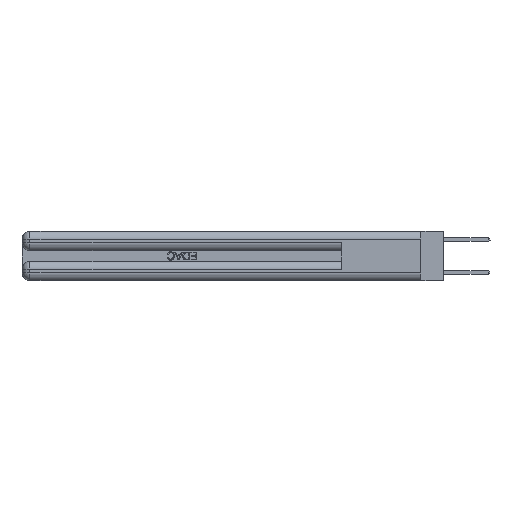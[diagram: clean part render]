
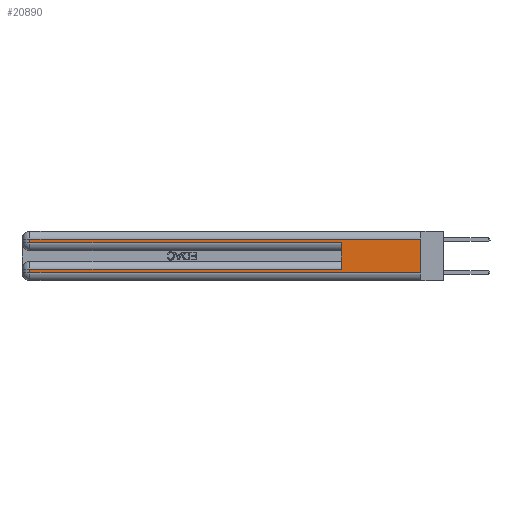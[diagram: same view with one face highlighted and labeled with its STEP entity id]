
A CAD part, left-side view. The second image highlights one B-rep face of the part: STEP entity #20890.
In plain terms, the highlighted planar face has unit normal (-1, 0, 0).
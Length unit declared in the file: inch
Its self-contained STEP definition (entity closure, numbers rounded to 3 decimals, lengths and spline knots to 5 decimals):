
#83 = LINE ( 'NONE', #20551, #28086 ) ;
#245 = LINE ( 'NONE', #5328, #17323 ) ;
#527 = CARTESIAN_POINT ( 'NONE',  ( 0., 2.94, 0.285 ) ) ;
#926 = DIRECTION ( 'NONE',  ( 0., 1., 0. ) ) ;
#1096 = DIRECTION ( 'NONE',  ( 0., -1., 0. ) ) ;
#1970 = EDGE_CURVE ( 'NONE', #8796, #6486, #13021, .T. ) ;
#2054 = ORIENTED_EDGE ( 'NONE', *, *, #26719, .F. ) ;
#3436 = LINE ( 'NONE', #9980, #7922 ) ;
#3776 = VECTOR ( 'NONE', #18258, 39.37008 ) ;
#4137 = CARTESIAN_POINT ( 'NONE',  ( 0., 2.94, 0.37 ) ) ;
#4388 = VERTEX_POINT ( 'NONE', #11405 ) ;
#5328 = CARTESIAN_POINT ( 'NONE',  ( 0., 0., 0.085 ) ) ;
#5373 = EDGE_CURVE ( 'NONE', #24988, #19430, #11162, .T. ) ;
#5878 = EDGE_LOOP ( 'NONE', ( #2054, #7955, #14554, #26247, #16652, #22531, #23214, #6233 ) ) ;
#6233 = ORIENTED_EDGE ( 'NONE', *, *, #23326, .T. ) ;
#6434 = CARTESIAN_POINT ( 'NONE',  ( 0., 2.94, 0.06 ) ) ;
#6486 = VERTEX_POINT ( 'NONE', #6434 ) ;
#6584 = DIRECTION ( 'NONE',  ( 0., -1., 0. ) ) ;
#6962 = CARTESIAN_POINT ( 'NONE',  ( 0., 0.6, 0.285 ) ) ;
#7140 = VECTOR ( 'NONE', #13058, 39.37008 ) ;
#7870 = CARTESIAN_POINT ( 'NONE',  ( 0., 2.94, 0.085 ) ) ;
#7922 = VECTOR ( 'NONE', #1096, 39.37008 ) ;
#7955 = ORIENTED_EDGE ( 'NONE', *, *, #17307, .T. ) ;
#8042 = PLANE ( 'NONE',  #15683 ) ;
#8404 = FACE_OUTER_BOUND ( 'NONE', #5878, .T. ) ;
#8779 = CARTESIAN_POINT ( 'NONE',  ( 0., 0., 0.06 ) ) ;
#8796 = VERTEX_POINT ( 'NONE', #7870 ) ;
#9980 = CARTESIAN_POINT ( 'NONE',  ( 0., 0., 0.06 ) ) ;
#10107 = VECTOR ( 'NONE', #6584, 39.37008 ) ;
#10286 = DIRECTION ( 'NONE',  ( 1., 0., 0. ) ) ;
#11162 = LINE ( 'NONE', #17073, #27997 ) ;
#11405 = CARTESIAN_POINT ( 'NONE',  ( 0., 0.6, 0.085 ) ) ;
#12168 = DIRECTION ( 'NONE',  ( 0., 0., 1. ) ) ;
#13021 = LINE ( 'NONE', #4137, #7140 ) ;
#13058 = DIRECTION ( 'NONE',  ( 0., 0., -1. ) ) ;
#13238 = VERTEX_POINT ( 'NONE', #6962 ) ;
#14554 = ORIENTED_EDGE ( 'NONE', *, *, #5373, .T. ) ;
#14805 = CARTESIAN_POINT ( 'NONE',  ( 0., 2.94, 0.31 ) ) ;
#15111 = EDGE_CURVE ( 'NONE', #4388, #13238, #27693, .T. ) ;
#15683 = AXIS2_PLACEMENT_3D ( 'NONE', #25625, #10286, #25714 ) ;
#16011 = CARTESIAN_POINT ( 'NONE',  ( 0., 0., 0.31 ) ) ;
#16053 = EDGE_CURVE ( 'NONE', #19430, #13238, #21203, .T. ) ;
#16280 = LINE ( 'NONE', #16011, #3776 ) ;
#16652 = ORIENTED_EDGE ( 'NONE', *, *, #15111, .F. ) ;
#17073 = CARTESIAN_POINT ( 'NONE',  ( 0., 2.94, 0.37 ) ) ;
#17307 = EDGE_CURVE ( 'NONE', #27368, #24988, #16280, .T. ) ;
#17323 = VECTOR ( 'NONE', #926, 39.37008 ) ;
#17467 = EDGE_CURVE ( 'NONE', #4388, #8796, #245, .T. ) ;
#18258 = DIRECTION ( 'NONE',  ( 0., 1., 0. ) ) ;
#18323 = DIRECTION ( 'NONE',  ( 0., 0., -1. ) ) ;
#18769 = CARTESIAN_POINT ( 'NONE',  ( 0., 0.6, 0.145 ) ) ;
#19430 = VERTEX_POINT ( 'NONE', #527 ) ;
#19864 = CARTESIAN_POINT ( 'NONE',  ( 0., 0., 0.285 ) ) ;
#19926 = VERTEX_POINT ( 'NONE', #8779 ) ;
#20551 = CARTESIAN_POINT ( 'NONE',  ( 0., 0., 0.37 ) ) ;
#20890 = ADVANCED_FACE ( 'NONE', ( #8404 ), #8042, .F. ) ;
#21203 = LINE ( 'NONE', #19864, #10107 ) ;
#22531 = ORIENTED_EDGE ( 'NONE', *, *, #17467, .T. ) ;
#22899 = CARTESIAN_POINT ( 'NONE',  ( 0., 0., 0.31 ) ) ;
#23214 = ORIENTED_EDGE ( 'NONE', *, *, #1970, .T. ) ;
#23326 = EDGE_CURVE ( 'NONE', #6486, #19926, #3436, .T. ) ;
#24988 = VERTEX_POINT ( 'NONE', #14805 ) ;
#25625 = CARTESIAN_POINT ( 'NONE',  ( 0., 0., 0.37 ) ) ;
#25714 = DIRECTION ( 'NONE',  ( 0., 0., -1. ) ) ;
#25885 = DIRECTION ( 'NONE',  ( 0., 0., -1. ) ) ;
#26247 = ORIENTED_EDGE ( 'NONE', *, *, #16053, .T. ) ;
#26345 = VECTOR ( 'NONE', #12168, 39.37008 ) ;
#26719 = EDGE_CURVE ( 'NONE', #27368, #19926, #83, .T. ) ;
#27368 = VERTEX_POINT ( 'NONE', #22899 ) ;
#27693 = LINE ( 'NONE', #18769, #26345 ) ;
#27997 = VECTOR ( 'NONE', #25885, 39.37008 ) ;
#28086 = VECTOR ( 'NONE', #18323, 39.37008 ) ;
